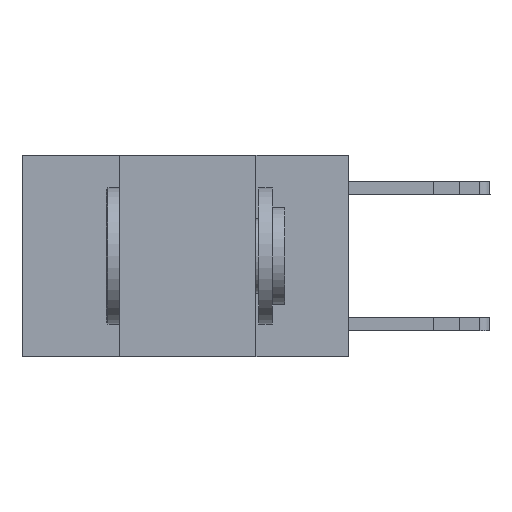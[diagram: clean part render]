
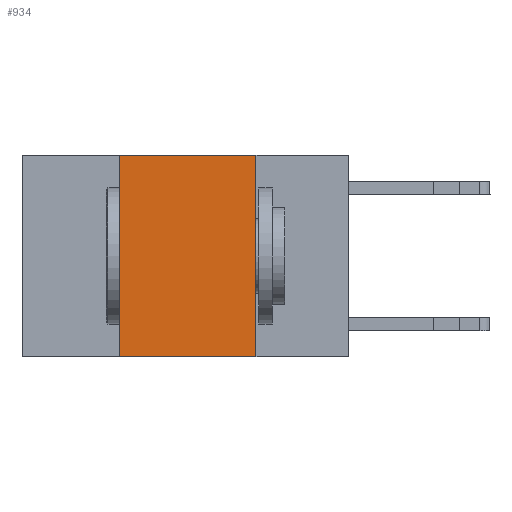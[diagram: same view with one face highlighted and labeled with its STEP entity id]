
A CAD part, left-side view. The second image highlights one B-rep face of the part: STEP entity #934.
In plain terms, the highlighted planar face has unit normal (-1, 0, 0).
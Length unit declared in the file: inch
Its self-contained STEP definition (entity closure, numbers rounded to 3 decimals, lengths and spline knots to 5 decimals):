
#759 = VECTOR ( 'NONE', #7545, 39.37008 ) ;
#934 = ADVANCED_FACE ( 'NONE', ( #17353 ), #7474, .F. ) ;
#1166 = CARTESIAN_POINT ( 'NONE',  ( 0., 0.6, 0. ) ) ;
#2645 = DIRECTION ( 'NONE',  ( 0., -1., 0. ) ) ;
#3031 = CARTESIAN_POINT ( 'NONE',  ( 0., 0.6, -0.37 ) ) ;
#3173 = EDGE_CURVE ( 'NONE', #8141, #3264, #15893, .T. ) ;
#3264 = VERTEX_POINT ( 'NONE', #10664 ) ;
#5317 = VECTOR ( 'NONE', #12756, 39.37008 ) ;
#6285 = EDGE_CURVE ( 'NONE', #3264, #16501, #10393, .T. ) ;
#6412 = CARTESIAN_POINT ( 'NONE',  ( 0., 0.42, -0.37 ) ) ;
#6614 = LINE ( 'NONE', #3031, #18170 ) ;
#7474 = PLANE ( 'NONE',  #9494 ) ;
#7545 = DIRECTION ( 'NONE',  ( 0., 0., 1. ) ) ;
#7716 = ORIENTED_EDGE ( 'NONE', *, *, #16430, .F. ) ;
#8141 = VERTEX_POINT ( 'NONE', #6412 ) ;
#8295 = EDGE_LOOP ( 'NONE', ( #7716, #8607, #12475, #12899 ) ) ;
#8607 = ORIENTED_EDGE ( 'NONE', *, *, #6285, .F. ) ;
#9140 = LINE ( 'NONE', #14096, #5317 ) ;
#9494 = AXIS2_PLACEMENT_3D ( 'NONE', #12107, #14355, #15503 ) ;
#10393 = LINE ( 'NONE', #1166, #17703 ) ;
#10664 = CARTESIAN_POINT ( 'NONE',  ( 0., 0.42, 0. ) ) ;
#12107 = CARTESIAN_POINT ( 'NONE',  ( 0., 0.6, 0. ) ) ;
#12299 = EDGE_CURVE ( 'NONE', #8141, #18227, #6614, .T. ) ;
#12475 = ORIENTED_EDGE ( 'NONE', *, *, #3173, .F. ) ;
#12756 = DIRECTION ( 'NONE',  ( 0., 0., -1. ) ) ;
#12899 = ORIENTED_EDGE ( 'NONE', *, *, #12299, .T. ) ;
#13071 = DIRECTION ( 'NONE',  ( 0., -1., 0. ) ) ;
#14096 = CARTESIAN_POINT ( 'NONE',  ( 0., 0.17, 0. ) ) ;
#14265 = CARTESIAN_POINT ( 'NONE',  ( 0., 0.17, 0. ) ) ;
#14355 = DIRECTION ( 'NONE',  ( 1., 0., 0. ) ) ;
#15503 = DIRECTION ( 'NONE',  ( 0., 0., -1. ) ) ;
#15893 = LINE ( 'NONE', #15980, #759 ) ;
#15980 = CARTESIAN_POINT ( 'NONE',  ( 0., 0.42, 0. ) ) ;
#16430 = EDGE_CURVE ( 'NONE', #16501, #18227, #9140, .T. ) ;
#16501 = VERTEX_POINT ( 'NONE', #14265 ) ;
#17353 = FACE_OUTER_BOUND ( 'NONE', #8295, .T. ) ;
#17703 = VECTOR ( 'NONE', #2645, 39.37008 ) ;
#18170 = VECTOR ( 'NONE', #13071, 39.37008 ) ;
#18192 = CARTESIAN_POINT ( 'NONE',  ( 0., 0.17, -0.37 ) ) ;
#18227 = VERTEX_POINT ( 'NONE', #18192 ) ;
